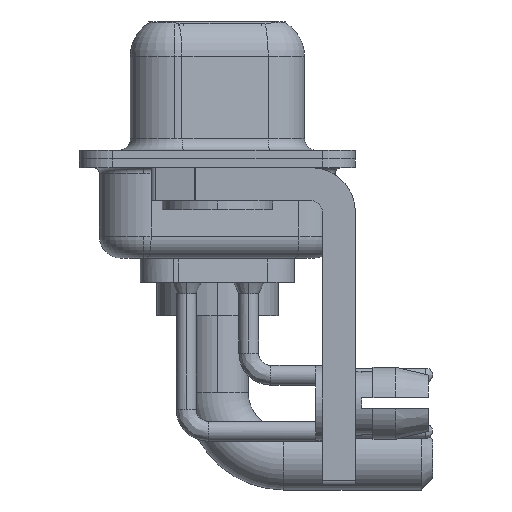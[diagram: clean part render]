
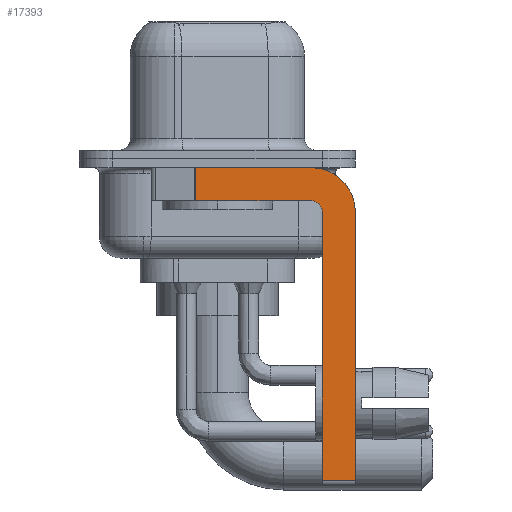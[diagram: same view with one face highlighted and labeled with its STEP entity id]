
A CAD part, left-side view. The second image highlights one B-rep face of the part: STEP entity #17393.
In plain terms, the highlighted planar face has unit normal (-1, 0, 0).
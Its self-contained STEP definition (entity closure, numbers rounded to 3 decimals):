
#161 = AXIS2_PLACEMENT_3D ( 'NONE', #12588, #19108, #2905 ) ;
#496 = CARTESIAN_POINT ( 'NONE',  ( -2.9, -4.75, -14.55 ) ) ;
#1088 = LINE ( 'NONE', #7564, #10629 ) ;
#1181 = CIRCLE ( 'NONE', #161, 2. ) ;
#1301 = DIRECTION ( 'NONE',  ( 0., 0., -1. ) ) ;
#1410 = DIRECTION ( 'NONE',  ( 0., -1., 0. ) ) ;
#1629 = CARTESIAN_POINT ( 'NONE',  ( -2.9, -6.25, -2.4 ) ) ;
#2249 = ORIENTED_EDGE ( 'NONE', *, *, #3431, .F. ) ;
#2805 = CIRCLE ( 'NONE', #13001, 0.5 ) ;
#2868 = VECTOR ( 'NONE', #19733, 1000. ) ;
#2905 = DIRECTION ( 'NONE',  ( 0., 0., -1. ) ) ;
#3030 = LINE ( 'NONE', #12617, #14908 ) ;
#3048 = EDGE_CURVE ( 'NONE', #10405, #15665, #17946, .T. ) ;
#3431 = EDGE_CURVE ( 'NONE', #5496, #18334, #2805, .T. ) ;
#4348 = LINE ( 'NONE', #17241, #15959 ) ;
#4852 = DIRECTION ( 'NONE',  ( 0., 0., -1. ) ) ;
#4968 = VERTEX_POINT ( 'NONE', #13630 ) ;
#5415 = ORIENTED_EDGE ( 'NONE', *, *, #16579, .F. ) ;
#5496 = VERTEX_POINT ( 'NONE', #15483 ) ;
#6095 = ORIENTED_EDGE ( 'NONE', *, *, #15269, .F. ) ;
#6437 = DIRECTION ( 'NONE',  ( 1., 0., 0. ) ) ;
#7367 = EDGE_LOOP ( 'NONE', ( #5415, #19508, #20162, #2249, #6095, #16313, #14197, #8285 ) ) ;
#7444 = DIRECTION ( 'NONE',  ( -1., 0., 0. ) ) ;
#7564 = CARTESIAN_POINT ( 'NONE',  ( -2.9, 0.978, -1.9 ) ) ;
#8285 = ORIENTED_EDGE ( 'NONE', *, *, #9706, .F. ) ;
#8384 = CARTESIAN_POINT ( 'NONE',  ( -2.9, -6.25, -2.4 ) ) ;
#8514 = CARTESIAN_POINT ( 'NONE',  ( -2.9, -4.25, -14.55 ) ) ;
#9706 = EDGE_CURVE ( 'NONE', #12818, #10405, #1181, .T. ) ;
#9715 = LINE ( 'NONE', #16116, #12944 ) ;
#9911 = EDGE_CURVE ( 'NONE', #12372, #15665, #19822, .T. ) ;
#10152 = CARTESIAN_POINT ( 'NONE',  ( -2.9, -4.25, -0.4 ) ) ;
#10405 = VERTEX_POINT ( 'NONE', #8384 ) ;
#10629 = VECTOR ( 'NONE', #1301, 1000. ) ;
#10735 = DIRECTION ( 'NONE',  ( 0., 0., 1. ) ) ;
#12262 = AXIS2_PLACEMENT_3D ( 'NONE', #16565, #6437, #4852 ) ;
#12372 = VERTEX_POINT ( 'NONE', #496 ) ;
#12588 = CARTESIAN_POINT ( 'NONE',  ( -2.9, -4.25, -2.4 ) ) ;
#12617 = CARTESIAN_POINT ( 'NONE',  ( -2.9, -4.25, -1.9 ) ) ;
#12818 = VERTEX_POINT ( 'NONE', #10152 ) ;
#12944 = VECTOR ( 'NONE', #1410, 1000. ) ;
#13001 = AXIS2_PLACEMENT_3D ( 'NONE', #14196, #7444, #17391 ) ;
#13630 = CARTESIAN_POINT ( 'NONE',  ( -2.9, 0.978, -1.9 ) ) ;
#13856 = EDGE_CURVE ( 'NONE', #18334, #4968, #3030, .T. ) ;
#14132 = VECTOR ( 'NONE', #16844, 1000. ) ;
#14196 = CARTESIAN_POINT ( 'NONE',  ( -2.9, -4.25, -2.4 ) ) ;
#14197 = ORIENTED_EDGE ( 'NONE', *, *, #3048, .F. ) ;
#14521 = VERTEX_POINT ( 'NONE', #16631 ) ;
#14908 = VECTOR ( 'NONE', #20618, 1000. ) ;
#15269 = EDGE_CURVE ( 'NONE', #12372, #5496, #4348, .T. ) ;
#15483 = CARTESIAN_POINT ( 'NONE',  ( -2.9, -4.75, -2.4 ) ) ;
#15665 = VERTEX_POINT ( 'NONE', #20756 ) ;
#15959 = VECTOR ( 'NONE', #10735, 1000. ) ;
#16116 = CARTESIAN_POINT ( 'NONE',  ( -2.9, 3., -0.4 ) ) ;
#16313 = ORIENTED_EDGE ( 'NONE', *, *, #9911, .T. ) ;
#16565 = CARTESIAN_POINT ( 'NONE',  ( -2.9, -4.25, -2.4 ) ) ;
#16579 = EDGE_CURVE ( 'NONE', #14521, #12818, #9715, .T. ) ;
#16631 = CARTESIAN_POINT ( 'NONE',  ( -2.9, 0.978, -0.4 ) ) ;
#16844 = DIRECTION ( 'NONE',  ( 0., -1., 0. ) ) ;
#17241 = CARTESIAN_POINT ( 'NONE',  ( -2.9, -4.75, -14.8 ) ) ;
#17391 = DIRECTION ( 'NONE',  ( 0., 0., 1. ) ) ;
#17393 = ADVANCED_FACE ( 'NONE', ( #20836 ), #18175, .F. ) ;
#17946 = LINE ( 'NONE', #1629, #2868 ) ;
#18175 = PLANE ( 'NONE',  #12262 ) ;
#18334 = VERTEX_POINT ( 'NONE', #20991 ) ;
#19108 = DIRECTION ( 'NONE',  ( 1., 0., 0. ) ) ;
#19508 = ORIENTED_EDGE ( 'NONE', *, *, #20964, .T. ) ;
#19733 = DIRECTION ( 'NONE',  ( 0., 0., -1. ) ) ;
#19822 = LINE ( 'NONE', #8514, #14132 ) ;
#20162 = ORIENTED_EDGE ( 'NONE', *, *, #13856, .F. ) ;
#20618 = DIRECTION ( 'NONE',  ( 0., 1., 0. ) ) ;
#20756 = CARTESIAN_POINT ( 'NONE',  ( -2.9, -6.25, -14.55 ) ) ;
#20836 = FACE_OUTER_BOUND ( 'NONE', #7367, .T. ) ;
#20964 = EDGE_CURVE ( 'NONE', #14521, #4968, #1088, .T. ) ;
#20991 = CARTESIAN_POINT ( 'NONE',  ( -2.9, -4.25, -1.9 ) ) ;
